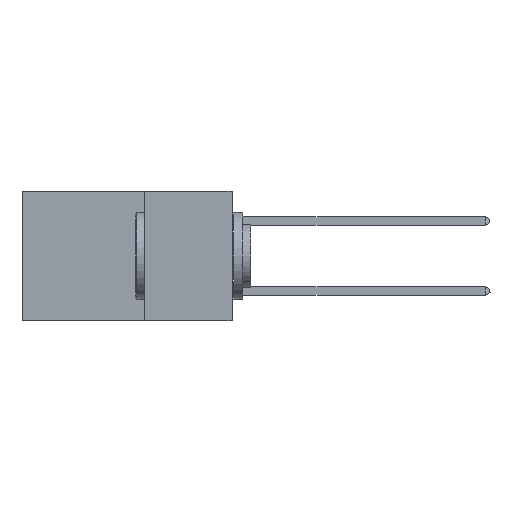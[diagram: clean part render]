
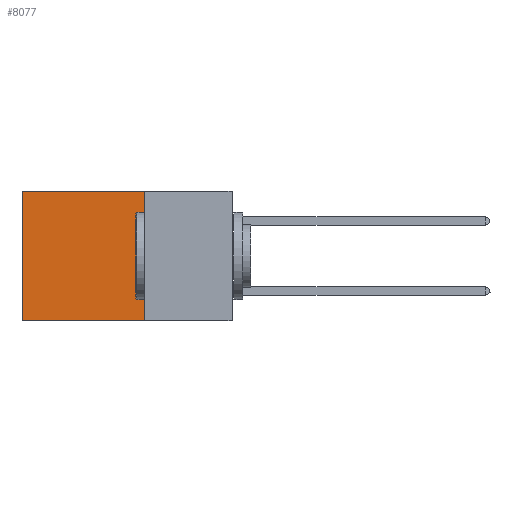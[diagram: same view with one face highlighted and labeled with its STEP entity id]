
A CAD part, left-side view. The second image highlights one B-rep face of the part: STEP entity #8077.
In plain terms, the highlighted planar face has unit normal (-1, 0, 0).
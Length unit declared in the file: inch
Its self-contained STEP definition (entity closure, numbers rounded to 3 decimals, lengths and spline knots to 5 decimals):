
#310 = VERTEX_POINT ( 'NONE', #29915 ) ;
#1392 = PLANE ( 'NONE',  #9991 ) ;
#1490 = VECTOR ( 'NONE', #28720, 39.37008 ) ;
#3313 = EDGE_CURVE ( 'NONE', #34775, #23189, #18002, .T. ) ;
#3446 = EDGE_LOOP ( 'NONE', ( #36720, #22777, #33333, #40918 ) ) ;
#3504 = VECTOR ( 'NONE', #17315, 39.37008 ) ;
#4032 = CARTESIAN_POINT ( 'NONE',  ( 0.2875, 0.6, 0. ) ) ;
#4281 = CARTESIAN_POINT ( 'NONE',  ( 0.2875, 0.25, -0.37 ) ) ;
#5480 = CARTESIAN_POINT ( 'NONE',  ( 0.2875, 0.6, 0. ) ) ;
#6781 = DIRECTION ( 'NONE',  ( 1., 0., 0. ) ) ;
#8077 = ADVANCED_FACE ( 'NONE', ( #28664 ), #1392, .F. ) ;
#8754 = CARTESIAN_POINT ( 'NONE',  ( 0.2875, 0.25, 0. ) ) ;
#9991 = AXIS2_PLACEMENT_3D ( 'NONE', #8754, #6781, #24921 ) ;
#17315 = DIRECTION ( 'NONE',  ( 0., 1., 0. ) ) ;
#18002 = LINE ( 'NONE', #5480, #1490 ) ;
#21067 = EDGE_CURVE ( 'NONE', #37767, #23189, #25476, .T. ) ;
#22777 = ORIENTED_EDGE ( 'NONE', *, *, #21067, .F. ) ;
#23189 = VERTEX_POINT ( 'NONE', #42565 ) ;
#23866 = VECTOR ( 'NONE', #34354, 39.37008 ) ;
#24258 = CARTESIAN_POINT ( 'NONE',  ( 0.2875, 0.25, 0. ) ) ;
#24921 = DIRECTION ( 'NONE',  ( 0., 0., -1. ) ) ;
#25476 = LINE ( 'NONE', #27652, #41059 ) ;
#27652 = CARTESIAN_POINT ( 'NONE',  ( 0.2875, 0.25, -0.37 ) ) ;
#28664 = FACE_OUTER_BOUND ( 'NONE', #3446, .T. ) ;
#28720 = DIRECTION ( 'NONE',  ( 0., 0., -1. ) ) ;
#29915 = CARTESIAN_POINT ( 'NONE',  ( 0.2875, 0.25, 0. ) ) ;
#30716 = CARTESIAN_POINT ( 'NONE',  ( 0.2875, 0.25, 0. ) ) ;
#31722 = EDGE_CURVE ( 'NONE', #310, #37767, #42012, .T. ) ;
#33333 = ORIENTED_EDGE ( 'NONE', *, *, #31722, .F. ) ;
#34001 = LINE ( 'NONE', #24258, #3504 ) ;
#34354 = DIRECTION ( 'NONE',  ( 0., 0., -1. ) ) ;
#34413 = DIRECTION ( 'NONE',  ( 0., 1., 0. ) ) ;
#34775 = VERTEX_POINT ( 'NONE', #4032 ) ;
#34813 = EDGE_CURVE ( 'NONE', #310, #34775, #34001, .T. ) ;
#36720 = ORIENTED_EDGE ( 'NONE', *, *, #3313, .T. ) ;
#37767 = VERTEX_POINT ( 'NONE', #4281 ) ;
#40918 = ORIENTED_EDGE ( 'NONE', *, *, #34813, .T. ) ;
#41059 = VECTOR ( 'NONE', #34413, 39.37008 ) ;
#42012 = LINE ( 'NONE', #30716, #23866 ) ;
#42565 = CARTESIAN_POINT ( 'NONE',  ( 0.2875, 0.6, -0.37 ) ) ;
